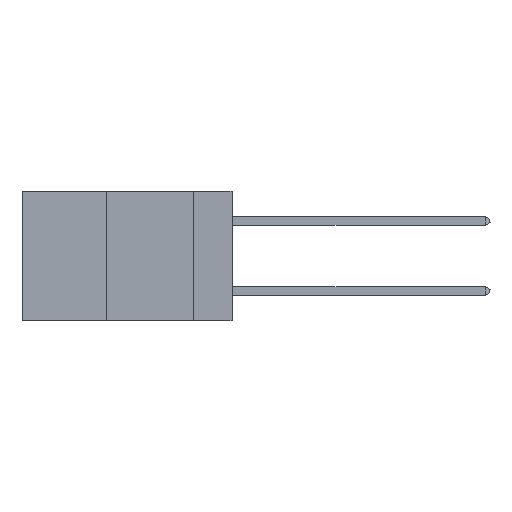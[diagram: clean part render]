
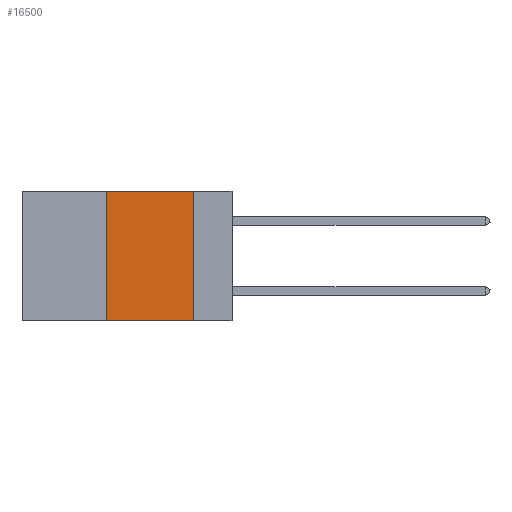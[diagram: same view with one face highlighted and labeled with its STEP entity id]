
A CAD part, left-side view. The second image highlights one B-rep face of the part: STEP entity #16500.
In plain terms, the highlighted planar face has unit normal (-1, 0, 0).
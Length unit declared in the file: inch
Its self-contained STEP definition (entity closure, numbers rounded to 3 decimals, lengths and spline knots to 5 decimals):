
#323 = CARTESIAN_POINT ( 'NONE',  ( 0., 0.11, 0. ) ) ;
#370 = VERTEX_POINT ( 'NONE', #9682 ) ;
#853 = DIRECTION ( 'NONE',  ( 0., 0., 1. ) ) ;
#1302 = DIRECTION ( 'NONE',  ( 0., 0., -1. ) ) ;
#1378 = EDGE_LOOP ( 'NONE', ( #14009, #1580, #11855, #1995 ) ) ;
#1550 = DIRECTION ( 'NONE',  ( 1., 0., 0. ) ) ;
#1580 = ORIENTED_EDGE ( 'NONE', *, *, #6632, .F. ) ;
#1751 = VECTOR ( 'NONE', #10373, 39.37008 ) ;
#1995 = ORIENTED_EDGE ( 'NONE', *, *, #12799, .T. ) ;
#5773 = LINE ( 'NONE', #8660, #10394 ) ;
#6492 = AXIS2_PLACEMENT_3D ( 'NONE', #6734, #1550, #10593 ) ;
#6632 = EDGE_CURVE ( 'NONE', #9397, #9812, #14452, .T. ) ;
#6734 = CARTESIAN_POINT ( 'NONE',  ( 0., 0.6, 0. ) ) ;
#6741 = CARTESIAN_POINT ( 'NONE',  ( 0., 0.11, -0.37 ) ) ;
#7240 = CARTESIAN_POINT ( 'NONE',  ( 0., 0.36, 0. ) ) ;
#7500 = CARTESIAN_POINT ( 'NONE',  ( 0., 0.6, 0. ) ) ;
#8485 = VERTEX_POINT ( 'NONE', #6741 ) ;
#8660 = CARTESIAN_POINT ( 'NONE',  ( 0., 0.36, 0. ) ) ;
#8677 = LINE ( 'NONE', #9114, #1751 ) ;
#9053 = EDGE_CURVE ( 'NONE', #9812, #8485, #10652, .T. ) ;
#9114 = CARTESIAN_POINT ( 'NONE',  ( 0., 0.6, -0.37 ) ) ;
#9331 = PLANE ( 'NONE',  #6492 ) ;
#9397 = VERTEX_POINT ( 'NONE', #7240 ) ;
#9682 = CARTESIAN_POINT ( 'NONE',  ( 0., 0.36, -0.37 ) ) ;
#9812 = VERTEX_POINT ( 'NONE', #323 ) ;
#10373 = DIRECTION ( 'NONE',  ( 0., -1., 0. ) ) ;
#10394 = VECTOR ( 'NONE', #853, 39.37008 ) ;
#10593 = DIRECTION ( 'NONE',  ( 0., 0., -1. ) ) ;
#10652 = LINE ( 'NONE', #12889, #16138 ) ;
#11855 = ORIENTED_EDGE ( 'NONE', *, *, #14938, .F. ) ;
#12799 = EDGE_CURVE ( 'NONE', #370, #8485, #8677, .T. ) ;
#12889 = CARTESIAN_POINT ( 'NONE',  ( 0., 0.11, 0. ) ) ;
#14009 = ORIENTED_EDGE ( 'NONE', *, *, #9053, .F. ) ;
#14067 = VECTOR ( 'NONE', #16301, 39.37008 ) ;
#14452 = LINE ( 'NONE', #7500, #14067 ) ;
#14938 = EDGE_CURVE ( 'NONE', #370, #9397, #5773, .T. ) ;
#16138 = VECTOR ( 'NONE', #1302, 39.37008 ) ;
#16301 = DIRECTION ( 'NONE',  ( 0., -1., 0. ) ) ;
#16411 = FACE_OUTER_BOUND ( 'NONE', #1378, .T. ) ;
#16500 = ADVANCED_FACE ( 'NONE', ( #16411 ), #9331, .F. ) ;
